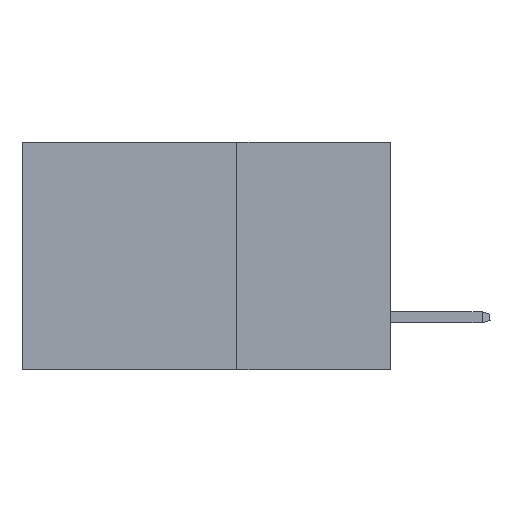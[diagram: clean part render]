
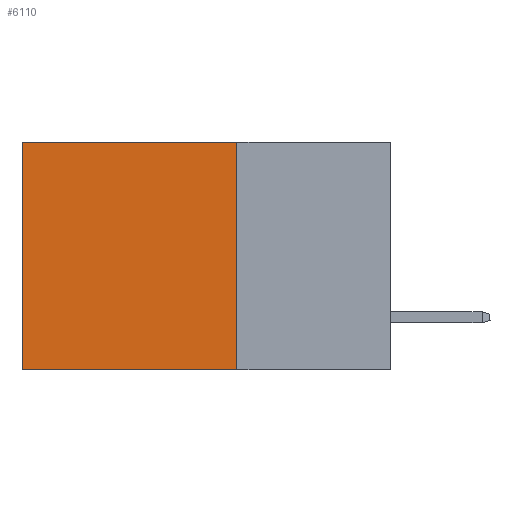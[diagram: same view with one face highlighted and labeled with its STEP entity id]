
A CAD part, left-side view. The second image highlights one B-rep face of the part: STEP entity #6110.
In plain terms, the highlighted planar face has unit normal (-1, 0, 0).
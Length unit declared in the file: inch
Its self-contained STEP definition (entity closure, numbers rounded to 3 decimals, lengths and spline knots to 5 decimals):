
#24 = CARTESIAN_POINT ( 'NONE',  ( 0.2875, 0.6, 0. ) ) ;
#708 = VECTOR ( 'NONE', #18882, 39.37008 ) ;
#1653 = DIRECTION ( 'NONE',  ( 0., 0., -1. ) ) ;
#1720 = LINE ( 'NONE', #26438, #22721 ) ;
#2010 = EDGE_CURVE ( 'NONE', #29780, #21422, #16785, .T. ) ;
#2189 = DIRECTION ( 'NONE',  ( 1., 0., 0. ) ) ;
#2939 = VERTEX_POINT ( 'NONE', #5325 ) ;
#3227 = LINE ( 'NONE', #20940, #8847 ) ;
#5325 = CARTESIAN_POINT ( 'NONE',  ( 0.2875, 0.25, 0. ) ) ;
#6110 = ADVANCED_FACE ( 'NONE', ( #13691 ), #11406, .F. ) ;
#7222 = DIRECTION ( 'NONE',  ( 0., 0., -1. ) ) ;
#7442 = ORIENTED_EDGE ( 'NONE', *, *, #11987, .T. ) ;
#7459 = DIRECTION ( 'NONE',  ( 0., 1., 0. ) ) ;
#7560 = DIRECTION ( 'NONE',  ( 0., 1., 0. ) ) ;
#8847 = VECTOR ( 'NONE', #1653, 39.37008 ) ;
#11406 = PLANE ( 'NONE',  #14801 ) ;
#11987 = EDGE_CURVE ( 'NONE', #2939, #29780, #1720, .T. ) ;
#12007 = CARTESIAN_POINT ( 'NONE',  ( 0.2875, 0.6, 0. ) ) ;
#13691 = FACE_OUTER_BOUND ( 'NONE', #18266, .T. ) ;
#13715 = ORIENTED_EDGE ( 'NONE', *, *, #2010, .T. ) ;
#13819 = VERTEX_POINT ( 'NONE', #28464 ) ;
#14801 = AXIS2_PLACEMENT_3D ( 'NONE', #16526, #2189, #7222 ) ;
#16062 = ORIENTED_EDGE ( 'NONE', *, *, #24675, .F. ) ;
#16526 = CARTESIAN_POINT ( 'NONE',  ( 0.2875, 0.25, 0. ) ) ;
#16785 = LINE ( 'NONE', #24, #708 ) ;
#18266 = EDGE_LOOP ( 'NONE', ( #13715, #27789, #16062, #7442 ) ) ;
#18882 = DIRECTION ( 'NONE',  ( 0., 0., -1. ) ) ;
#20940 = CARTESIAN_POINT ( 'NONE',  ( 0.2875, 0.25, 0. ) ) ;
#21422 = VERTEX_POINT ( 'NONE', #22267 ) ;
#21954 = EDGE_CURVE ( 'NONE', #13819, #21422, #29683, .T. ) ;
#22267 = CARTESIAN_POINT ( 'NONE',  ( 0.2875, 0.6, -0.37 ) ) ;
#22721 = VECTOR ( 'NONE', #7459, 39.37008 ) ;
#22933 = VECTOR ( 'NONE', #7560, 39.37008 ) ;
#24220 = CARTESIAN_POINT ( 'NONE',  ( 0.2875, 0.25, -0.37 ) ) ;
#24675 = EDGE_CURVE ( 'NONE', #2939, #13819, #3227, .T. ) ;
#26438 = CARTESIAN_POINT ( 'NONE',  ( 0.2875, 0.25, 0. ) ) ;
#27789 = ORIENTED_EDGE ( 'NONE', *, *, #21954, .F. ) ;
#28464 = CARTESIAN_POINT ( 'NONE',  ( 0.2875, 0.25, -0.37 ) ) ;
#29683 = LINE ( 'NONE', #24220, #22933 ) ;
#29780 = VERTEX_POINT ( 'NONE', #12007 ) ;
